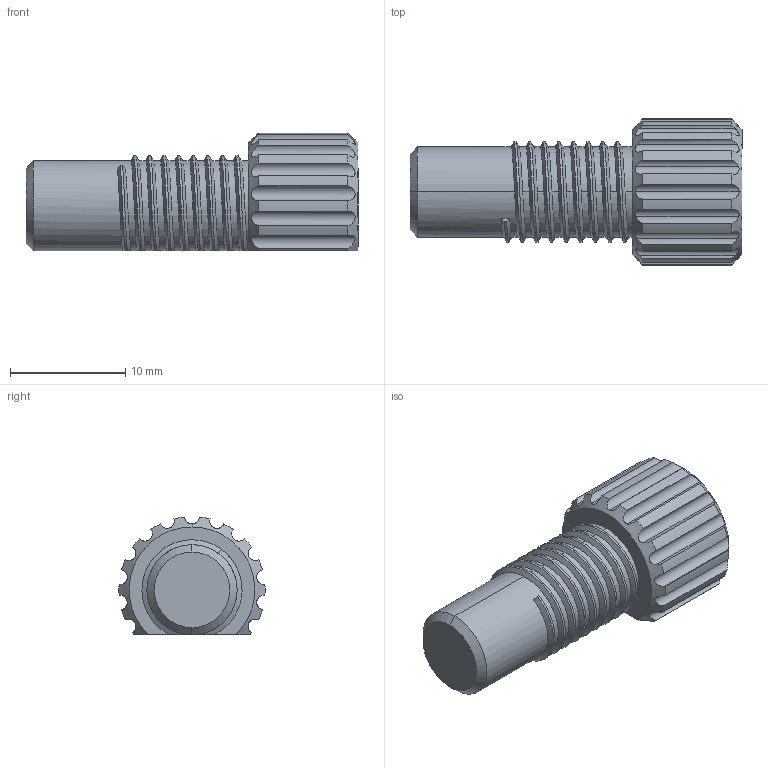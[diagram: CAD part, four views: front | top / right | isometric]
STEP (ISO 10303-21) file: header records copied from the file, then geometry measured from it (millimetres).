
FILE_DESCRIPTION (( 'STEP AP203' ), '1' );
FILE_NAME ('AF-WF-SS-PRT-002-STEP.STEP', '2020-07-22T00:01:18', ( '' ), ( '' ), 'SwSTEP 2.0', 'SolidWorks 2018', '' );
FILE_SCHEMA (( 'CONFIG_CONTROL_DESIGN' ));
Length unit declared in the file: inch
Products named in the file (1): AF-WF-SS-PRT-002-STEP
Bounding box: 28.83 x 12.7 x 10.24 mm (x, y, z)
Volume: 1901.8 mm3; surface area: 1232.6 mm2
Topology: 1 solids, 1 shells, 106 faces, 269 edges, 166 vertices
Faces by surface type: cylinder 57, bspline 27, plane 17, cone 5
Entity records: 11330 total; most frequent: CARTESIAN_POINT 9118, ORIENTED_EDGE 538, DIRECTION 333, EDGE_CURVE 269, VERTEX_POINT 166, AXIS2_PLACEMENT_3D 123, EDGE_LOOP 107, ADVANCED_FACE 106
